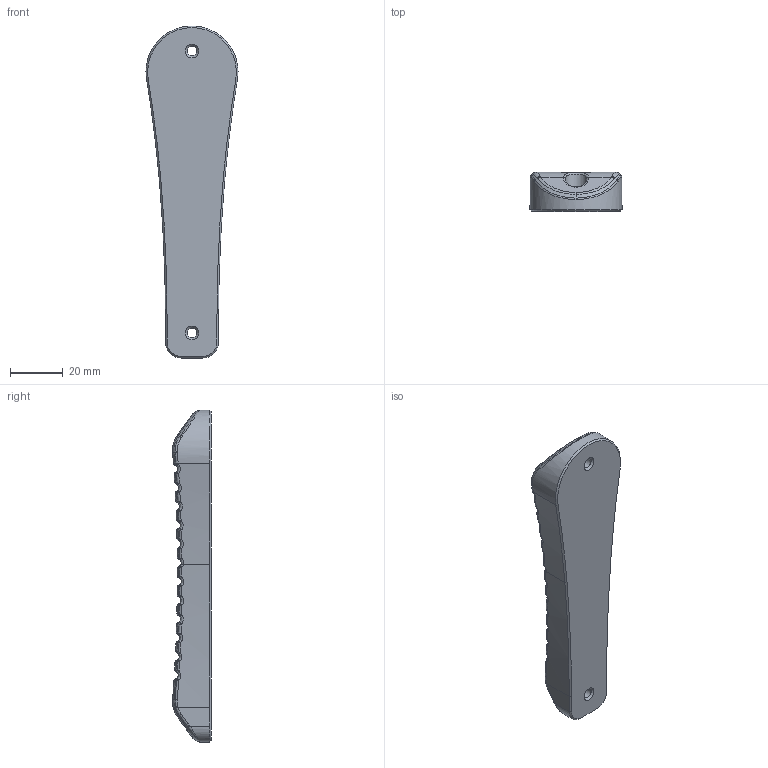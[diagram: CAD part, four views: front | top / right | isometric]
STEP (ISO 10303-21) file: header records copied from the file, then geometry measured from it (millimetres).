
FILE_DESCRIPTION(/* description */ (''),/* implementation_level */ '2;1');
FILE_NAME(/* name */ 'Buttpad.step',/* time_stamp */ '2021-08-21T08:40:12-04:00',/* author */ (''),/* organization */ (''),/* preprocessor_version */ 'ST-DEVELOPER v18.1',/* originating_system */ 'Autodesk Translation Framework v10.9.0.1377',/* authorisation */ '');
FILE_SCHEMA (('AUTOMOTIVE_DESIGN { 1 0 10303 214 3 1 1 }'));
Length unit declared in the file: millimetre
Products named in the file (1): Buttpad
Bounding box: 34.82 x 14.74 x 125.65 mm (x, y, z)
Volume: 38457.4 mm3; surface area: 10204.3 mm2
Topology: 1 solids, 1 shells, 431 faces, 1001 edges, 572 vertices
Faces by surface type: bspline 334, cylinder 68, plane 14, cone 11, torus 4
Full cylindrical faces by diameter (mm): 3.7 x2, 8 x2
Entity records: 18891 total; most frequent: CARTESIAN_POINT 11075, ORIENTED_EDGE 2002, EDGE_CURVE 1001, DIRECTION 934, VERTEX_POINT 572, B_SPLINE_CURVE_WITH_KNOTS 569, EDGE_LOOP 435, FACE_OUTER_BOUND 431
